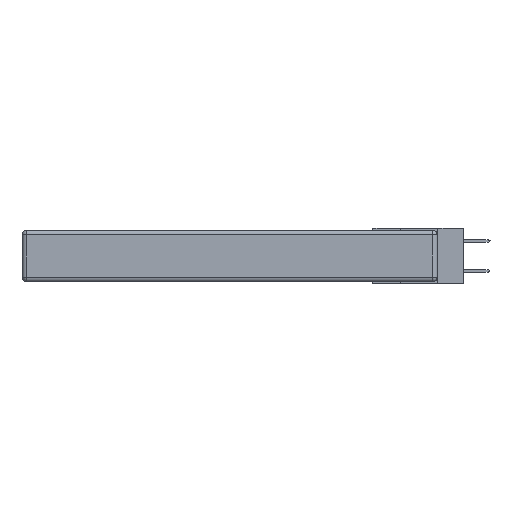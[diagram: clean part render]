
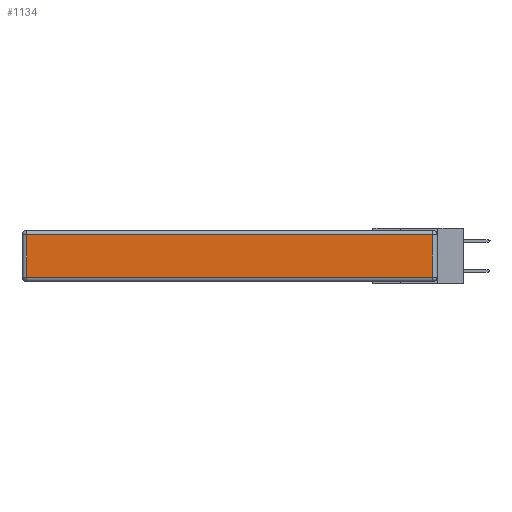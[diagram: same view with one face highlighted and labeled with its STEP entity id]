
A CAD part, left-side view. The second image highlights one B-rep face of the part: STEP entity #1134.
In plain terms, the highlighted planar face has unit normal (-1, 0, 0).
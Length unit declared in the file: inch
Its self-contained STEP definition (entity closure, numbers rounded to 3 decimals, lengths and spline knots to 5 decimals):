
#327 = CARTESIAN_POINT ( 'NONE',  ( 0., 0., -0.343 ) ) ;
#847 = ORIENTED_EDGE ( 'NONE', *, *, #22466, .T. ) ;
#1134 = ADVANCED_FACE ( 'NONE', ( #15559 ), #4840, .T. ) ;
#1309 = LINE ( 'NONE', #19389, #10573 ) ;
#1535 = VERTEX_POINT ( 'NONE', #3335 ) ;
#2008 = DIRECTION ( 'NONE',  ( 0., 1., 0. ) ) ;
#3335 = CARTESIAN_POINT ( 'NONE',  ( 0., 0.03, -0.313 ) ) ;
#3808 = VERTEX_POINT ( 'NONE', #19013 ) ;
#4750 = VERTEX_POINT ( 'NONE', #6059 ) ;
#4840 = PLANE ( 'NONE',  #28863 ) ;
#5127 = CARTESIAN_POINT ( 'NONE',  ( 0., 0.03, -0.343 ) ) ;
#6059 = CARTESIAN_POINT ( 'NONE',  ( 0., 2.72, -0.03 ) ) ;
#6288 = DIRECTION ( 'NONE',  ( 0., 0., -1. ) ) ;
#6891 = CARTESIAN_POINT ( 'NONE',  ( 0., 2.75, -0.03 ) ) ;
#7239 = DIRECTION ( 'NONE',  ( 0., 0., 1. ) ) ;
#7615 = ORIENTED_EDGE ( 'NONE', *, *, #29182, .T. ) ;
#8058 = VERTEX_POINT ( 'NONE', #29020 ) ;
#8319 = EDGE_LOOP ( 'NONE', ( #7615, #21186, #25756, #847 ) ) ;
#9520 = EDGE_CURVE ( 'NONE', #1535, #8058, #29930, .T. ) ;
#10573 = VECTOR ( 'NONE', #26397, 39.37008 ) ;
#12060 = VECTOR ( 'NONE', #17190, 39.37008 ) ;
#15559 = FACE_OUTER_BOUND ( 'NONE', #8319, .T. ) ;
#16497 = DIRECTION ( 'NONE',  ( -1., 0., 0. ) ) ;
#17190 = DIRECTION ( 'NONE',  ( 0., 0., 1. ) ) ;
#19013 = CARTESIAN_POINT ( 'NONE',  ( 0., 2.72, -0.313 ) ) ;
#19389 = CARTESIAN_POINT ( 'NONE',  ( 0., 0., -0.313 ) ) ;
#20296 = CARTESIAN_POINT ( 'NONE',  ( 0., 2.72, -0.343 ) ) ;
#21186 = ORIENTED_EDGE ( 'NONE', *, *, #9520, .T. ) ;
#21928 = LINE ( 'NONE', #20296, #23782 ) ;
#22466 = EDGE_CURVE ( 'NONE', #4750, #3808, #21928, .T. ) ;
#23664 = LINE ( 'NONE', #6891, #24019 ) ;
#23782 = VECTOR ( 'NONE', #6288, 39.37008 ) ;
#24019 = VECTOR ( 'NONE', #2008, 39.37008 ) ;
#25090 = EDGE_CURVE ( 'NONE', #8058, #4750, #23664, .T. ) ;
#25756 = ORIENTED_EDGE ( 'NONE', *, *, #25090, .T. ) ;
#26397 = DIRECTION ( 'NONE',  ( 0., -1., 0. ) ) ;
#28863 = AXIS2_PLACEMENT_3D ( 'NONE', #327, #16497, #7239 ) ;
#29020 = CARTESIAN_POINT ( 'NONE',  ( 0., 0.03, -0.03 ) ) ;
#29182 = EDGE_CURVE ( 'NONE', #3808, #1535, #1309, .T. ) ;
#29930 = LINE ( 'NONE', #5127, #12060 ) ;
